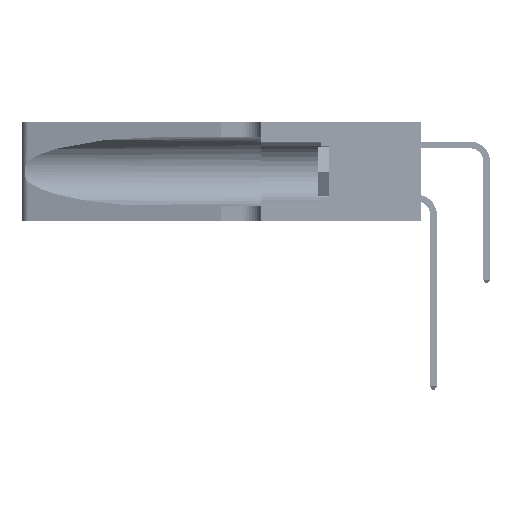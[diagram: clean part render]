
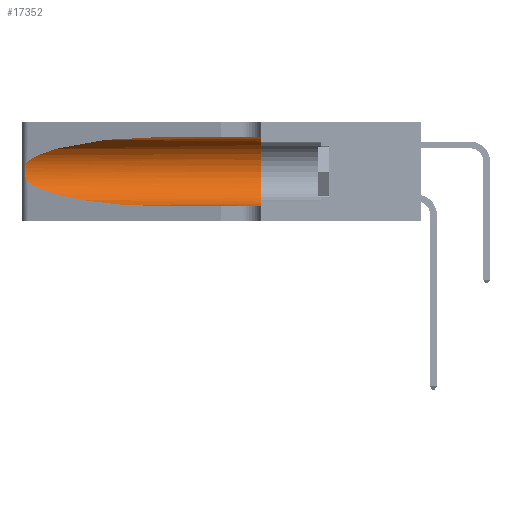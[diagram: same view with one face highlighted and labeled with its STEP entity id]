
A CAD part, left-side view. The second image highlights one B-rep face of the part: STEP entity #17352.
In plain terms, the highlighted cylindrical face has radius 3.308 mm (diameter 6.617 mm), a partial arc.
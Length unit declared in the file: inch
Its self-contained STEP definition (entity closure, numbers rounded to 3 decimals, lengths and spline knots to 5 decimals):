
#1444 = CARTESIAN_POINT ( 'NONE',  ( 0.1305, 0.72297, 0.05475 ) ) ;
#1889 = CARTESIAN_POINT ( 'NONE',  ( 0.26075, 1.23896, 0.19203 ) ) ;
#2853 = DIRECTION ( 'NONE',  ( 0., -1., 0. ) ) ;
#2991 = CARTESIAN_POINT ( 'NONE',  ( 0.2373, 1.15595, 0.28018 ) ) ;
#3116 = DIRECTION ( 'NONE',  ( 0., 0., 1. ) ) ;
#3362 = VERTEX_POINT ( 'NONE', #20685 ) ;
#4111 = CARTESIAN_POINT ( 'NONE',  ( 0.1305, 0.35, 0.31525 ) ) ;
#5320 = B_SPLINE_CURVE_WITH_KNOTS ( 'NONE', 3,
 ( #39560, #47793, #47959, #22841, #52167, #27067, #1889, #31285, #6108, #35527, #10318, #39724, #14546, #43940 ),
 .UNSPECIFIED., .F., .F.,
 ( 4, 2, 2, 2, 2, 2, 4 ),
 ( 0., 0.00027, 0.00053, 0.00107, 0.0016, 0.00187, 0.00214 ),
 .UNSPECIFIED. ) ;
#5784 = FACE_OUTER_BOUND ( 'NONE', #39554, .T. ) ;
#6108 = CARTESIAN_POINT ( 'NONE',  ( 0.26017, 1.23833, 0.17102 ) ) ;
#6109 = ORIENTED_EDGE ( 'NONE', *, *, #20920, .T. ) ;
#6836 = ORIENTED_EDGE ( 'NONE', *, *, #54010, .F. ) ;
#7973 = VECTOR ( 'NONE', #53192, 39.37008 ) ;
#8922 = ORIENTED_EDGE ( 'NONE', *, *, #41695, .T. ) ;
#9439 = ORIENTED_EDGE ( 'NONE', *, *, #27058, .F. ) ;
#10318 = CARTESIAN_POINT ( 'NONE',  ( 0.25789, 1.23486, 0.15765 ) ) ;
#10762 = EDGE_CURVE ( 'NONE', #21718, #3362, #32031, .T. ) ;
#11833 = VERTEX_POINT ( 'NONE', #48276 ) ;
#14546 = CARTESIAN_POINT ( 'NONE',  ( 0.25555, 1.22993, 0.14849 ) ) ;
#15276 = VERTEX_POINT ( 'NONE', #4111 ) ;
#17352 = ADVANCED_FACE ( 'NONE', ( #5784 ), #36704, .F. ) ;
#18124 = CARTESIAN_POINT ( 'NONE',  ( 0.18966, 0.96281, 0.05475 ) ) ;
#20685 = CARTESIAN_POINT ( 'NONE',  ( 0.1305, 0.35, 0.05475 ) ) ;
#20920 = EDGE_CURVE ( 'NONE', #38807, #21718, #41610, .T. ) ;
#21718 = VERTEX_POINT ( 'NONE', #32411 ) ;
#22812 = CARTESIAN_POINT ( 'NONE',  ( 0.1305, 1.61858, 0.05475 ) ) ;
#22841 = CARTESIAN_POINT ( 'NONE',  ( 0.25787, 1.23484, 0.2124 ) ) ;
#23970 = CARTESIAN_POINT ( 'NONE',  ( 0.1305, 0.72297, 0.31525 ) ) ;
#24104 = ORIENTED_EDGE ( 'NONE', *, *, #24904, .T. ) ;
#24904 = EDGE_CURVE ( 'NONE', #33625, #38807, #5320, .T. ) ;
#26608 = CARTESIAN_POINT ( 'NONE',  ( 0.25487, 1.22718, 0.14631 ) ) ;
#27058 = EDGE_CURVE ( 'NONE', #15276, #3362, #51508, .T. ) ;
#27067 = CARTESIAN_POINT ( 'NONE',  ( 0.26018, 1.23835, 0.19895 ) ) ;
#28175 = CARTESIAN_POINT ( 'NONE',  ( 0.18966, 0.96281, 0.31525 ) ) ;
#28290 = DIRECTION ( 'NONE',  ( 0., 1., 0. ) ) ;
#29429 = CARTESIAN_POINT ( 'NONE',  ( 0.25487, 1.22718, 0.22369 ) ) ;
#31285 = CARTESIAN_POINT ( 'NONE',  ( 0.26075, 1.23896, 0.178 ) ) ;
#32031 = LINE ( 'NONE', #22812, #54295 ) ;
#32253 = DIRECTION ( 'NONE',  ( 0., 0., -1. ) ) ;
#32403 = CARTESIAN_POINT ( 'NONE',  ( 0.25487, 1.22718, 0.22369 ) ) ;
#32411 = CARTESIAN_POINT ( 'NONE',  ( 0.1305, 0.72297, 0.05475 ) ) ;
#33625 = VERTEX_POINT ( 'NONE', #29429 ) ;
#35527 = CARTESIAN_POINT ( 'NONE',  ( 0.25856, 1.23593, 0.16098 ) ) ;
#35723 = CARTESIAN_POINT ( 'NONE',  ( 0.25487, 1.22718, 0.14631 ) ) ;
#36704 = CYLINDRICAL_SURFACE ( 'NONE', #52870, 0.13025 ) ;
#38807 = VERTEX_POINT ( 'NONE', #35723 ) ;
#39554 = EDGE_LOOP ( 'NONE', ( #8922, #24104, #6109, #41140, #9439, #6836 ) ) ;
#39560 = CARTESIAN_POINT ( 'NONE',  ( 0.25487, 1.22718, 0.22369 ) ) ;
#39724 = CARTESIAN_POINT ( 'NONE',  ( 0.25639, 1.23186, 0.15144 ) ) ;
#41140 = ORIENTED_EDGE ( 'NONE', *, *, #10762, .T. ) ;
#41519 = LINE ( 'NONE', #48991, #7973 ) ;
#41610 =( BOUNDED_CURVE ( )  B_SPLINE_CURVE ( 3, ( #26608, #47509, #18124, #1444 ),
 .UNSPECIFIED., .F., .T. ) 
 B_SPLINE_CURVE_WITH_KNOTS ( ( 4, 4 ),
 ( 3.44316, 4.71239 ),
 .UNSPECIFIED. ) 
 CURVE ( )  GEOMETRIC_REPRESENTATION_ITEM ( )  RATIONAL_B_SPLINE_CURVE ( ( 1., 0.87, 0.87, 1. ) ) 
 REPRESENTATION_ITEM ( '' )  );
#41695 = EDGE_CURVE ( 'NONE', #11833, #33625, #49831, .T. ) ;
#43940 = CARTESIAN_POINT ( 'NONE',  ( 0.25487, 1.22718, 0.14631 ) ) ;
#46202 = AXIS2_PLACEMENT_3D ( 'NONE', #53403, #28290, #3116 ) ;
#47509 = CARTESIAN_POINT ( 'NONE',  ( 0.2373, 1.15595, 0.08982 ) ) ;
#47793 = CARTESIAN_POINT ( 'NONE',  ( 0.25555, 1.22994, 0.2215 ) ) ;
#47929 = DIRECTION ( 'NONE',  ( 0., -1., 0. ) ) ;
#47959 = CARTESIAN_POINT ( 'NONE',  ( 0.25639, 1.23184, 0.21858 ) ) ;
#48276 = CARTESIAN_POINT ( 'NONE',  ( 0.1305, 0.72297, 0.31525 ) ) ;
#48924 = CARTESIAN_POINT ( 'NONE',  ( 0.1305, 1.61858, 0.185 ) ) ;
#48991 = CARTESIAN_POINT ( 'NONE',  ( 0.1305, 1.61858, 0.31525 ) ) ;
#49831 =( BOUNDED_CURVE ( )  B_SPLINE_CURVE ( 3, ( #23970, #28175, #2991, #32403 ),
 .UNSPECIFIED., .F., .T. ) 
 B_SPLINE_CURVE_WITH_KNOTS ( ( 4, 4 ),
 ( 1.5708, 2.84003 ),
 .UNSPECIFIED. ) 
 CURVE ( )  GEOMETRIC_REPRESENTATION_ITEM ( )  RATIONAL_B_SPLINE_CURVE ( ( 1., 0.87, 0.87, 1. ) ) 
 REPRESENTATION_ITEM ( '' )  );
#51508 = CIRCLE ( 'NONE', #46202, 0.13025 ) ;
#52167 = CARTESIAN_POINT ( 'NONE',  ( 0.25854, 1.2359, 0.20912 ) ) ;
#52870 = AXIS2_PLACEMENT_3D ( 'NONE', #48924, #2853, #32253 ) ;
#53192 = DIRECTION ( 'NONE',  ( 0., -1., 0. ) ) ;
#53403 = CARTESIAN_POINT ( 'NONE',  ( 0.1305, 0.35, 0.185 ) ) ;
#54010 = EDGE_CURVE ( 'NONE', #11833, #15276, #41519, .T. ) ;
#54295 = VECTOR ( 'NONE', #47929, 39.37008 ) ;
